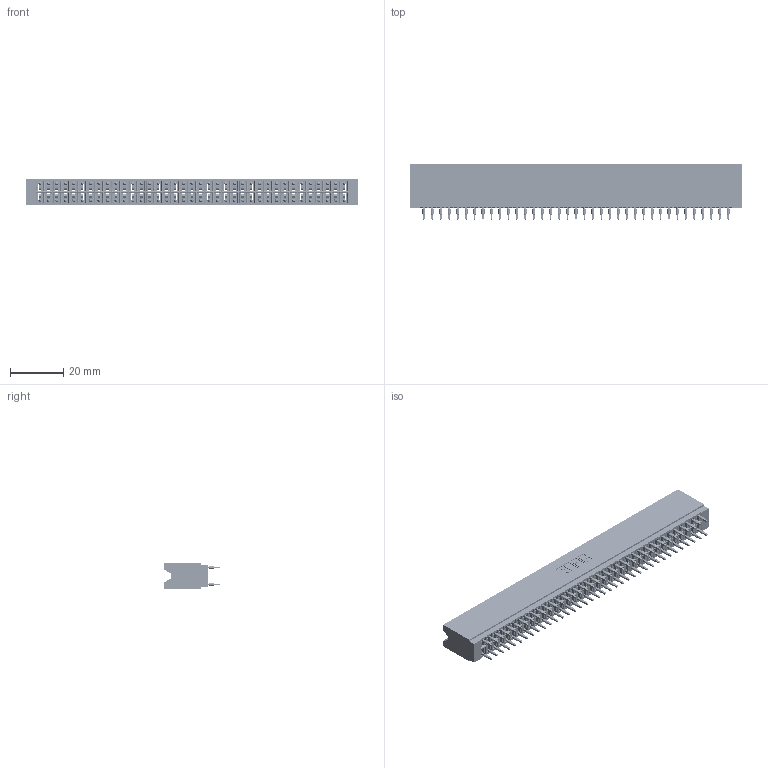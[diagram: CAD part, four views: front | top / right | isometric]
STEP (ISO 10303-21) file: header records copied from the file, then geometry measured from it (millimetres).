
FILE_DESCRIPTION (( 'STEP AP203' ), '1' );
FILE_NAME ('746-074-560-206.STEP', '2026-03-04T15:48:36', ( '' ), ( '' ), 'SwSTEP 2.0', 'SolidWorks 2023', '' );
FILE_SCHEMA (( 'CONFIG_CONTROL_DESIGN' ));
Length unit declared in the file: millimetre
Products named in the file (3): 746 Part_.515 Slot Depth - 06; 746-292-001_560; 746-074-560-206
Assembly tree (75 placements, depth 2):
  746-074-560-206
    746 Part_.515 Slot Depth - 06
    746-292-001_560  x74
Bounding box: 124.71 x 20.82 x 9.91 mm (x, y, z)
Volume: 13633.6 mm3; surface area: 23016.6 mm2
Topology: 75 solids, 75 shells, 7091 faces, 19727 edges, 12644 vertices
Faces by surface type: plane 3534, cylinder 1633, bspline 1480, torus 444
Entity records: 58010 total; most frequent: CARTESIAN_POINT 11572, ORIENTED_EDGE 9962, DIRECTION 8333, EDGE_CURVE 4981, LINE 4419, VECTOR 4419, VERTEX_POINT 3300, AXIS2_PLACEMENT_3D 1957
